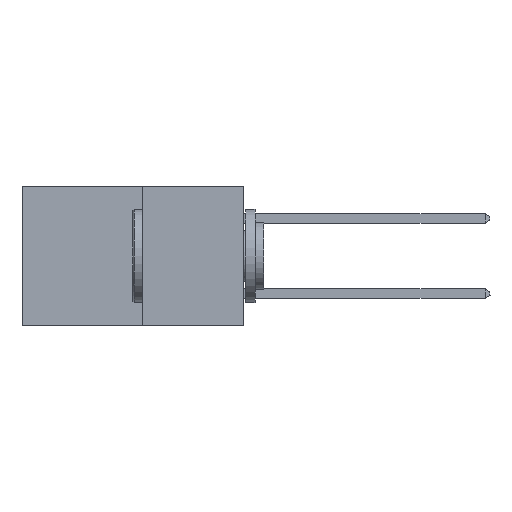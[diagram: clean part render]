
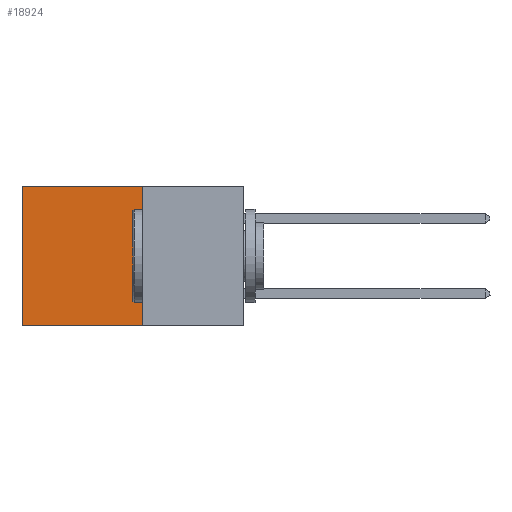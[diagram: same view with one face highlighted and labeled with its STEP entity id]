
A CAD part, left-side view. The second image highlights one B-rep face of the part: STEP entity #18924.
In plain terms, the highlighted planar face has unit normal (-1, 0, 0).
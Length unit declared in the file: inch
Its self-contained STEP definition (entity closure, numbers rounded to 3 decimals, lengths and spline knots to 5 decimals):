
#1253 = LINE ( 'NONE', #9834, #10235 ) ;
#1822 = ORIENTED_EDGE ( 'NONE', *, *, #18128, .T. ) ;
#2012 = ORIENTED_EDGE ( 'NONE', *, *, #8417, .F. ) ;
#2807 = DIRECTION ( 'NONE',  ( 0., 1., 0. ) ) ;
#2829 = CARTESIAN_POINT ( 'NONE',  ( 0.277, 0.27, -0.37 ) ) ;
#2983 = ORIENTED_EDGE ( 'NONE', *, *, #5224, .F. ) ;
#3106 = ORIENTED_EDGE ( 'NONE', *, *, #16501, .T. ) ;
#5224 = EDGE_CURVE ( 'NONE', #9027, #8839, #1253, .T. ) ;
#7241 = PLANE ( 'NONE',  #8497 ) ;
#7856 = CARTESIAN_POINT ( 'NONE',  ( 0.277, 0.27, 0. ) ) ;
#8214 = LINE ( 'NONE', #7856, #17606 ) ;
#8417 = EDGE_CURVE ( 'NONE', #8839, #18920, #15081, .T. ) ;
#8497 = AXIS2_PLACEMENT_3D ( 'NONE', #18490, #9117, #22322 ) ;
#8839 = VERTEX_POINT ( 'NONE', #19050 ) ;
#9027 = VERTEX_POINT ( 'NONE', #11049 ) ;
#9117 = DIRECTION ( 'NONE',  ( 1., 0., 0. ) ) ;
#9754 = DIRECTION ( 'NONE',  ( 0., 0., -1. ) ) ;
#9834 = CARTESIAN_POINT ( 'NONE',  ( 0.277, 0.27, -0.37 ) ) ;
#10232 = VERTEX_POINT ( 'NONE', #12105 ) ;
#10235 = VECTOR ( 'NONE', #9754, 39.37008 ) ;
#10661 = VECTOR ( 'NONE', #2807, 39.37008 ) ;
#11049 = CARTESIAN_POINT ( 'NONE',  ( 0.277, 0.27, 0. ) ) ;
#12105 = CARTESIAN_POINT ( 'NONE',  ( 0.277, 0.59, 0. ) ) ;
#12506 = DIRECTION ( 'NONE',  ( 0., 0., -1. ) ) ;
#13527 = DIRECTION ( 'NONE',  ( 0., 1., 0. ) ) ;
#15081 = LINE ( 'NONE', #2829, #10661 ) ;
#15417 = VECTOR ( 'NONE', #12506, 39.37008 ) ;
#16010 = LINE ( 'NONE', #20048, #15417 ) ;
#16501 = EDGE_CURVE ( 'NONE', #9027, #10232, #8214, .T. ) ;
#16592 = CARTESIAN_POINT ( 'NONE',  ( 0.277, 0.59, -0.37 ) ) ;
#17606 = VECTOR ( 'NONE', #13527, 39.37008 ) ;
#18128 = EDGE_CURVE ( 'NONE', #10232, #18920, #16010, .T. ) ;
#18303 = FACE_OUTER_BOUND ( 'NONE', #21760, .T. ) ;
#18490 = CARTESIAN_POINT ( 'NONE',  ( 0.277, 0.27, -0.37 ) ) ;
#18920 = VERTEX_POINT ( 'NONE', #16592 ) ;
#18924 = ADVANCED_FACE ( 'NONE', ( #18303 ), #7241, .F. ) ;
#19050 = CARTESIAN_POINT ( 'NONE',  ( 0.277, 0.27, -0.37 ) ) ;
#20048 = CARTESIAN_POINT ( 'NONE',  ( 0.277, 0.59, -0.37 ) ) ;
#21760 = EDGE_LOOP ( 'NONE', ( #1822, #2012, #2983, #3106 ) ) ;
#22322 = DIRECTION ( 'NONE',  ( 0., 0., -1. ) ) ;
